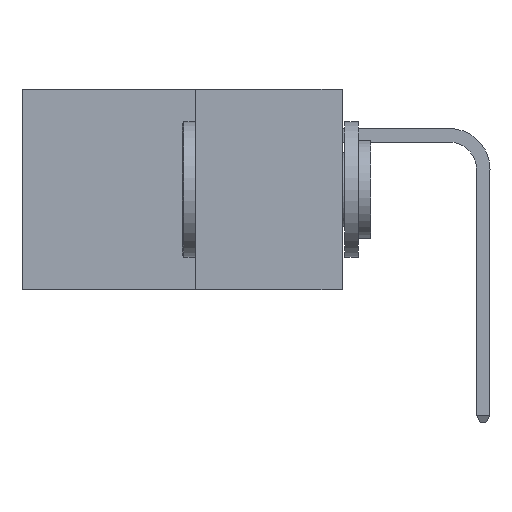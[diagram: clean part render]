
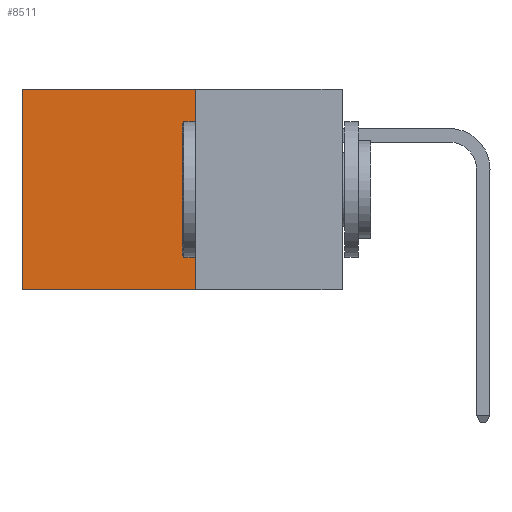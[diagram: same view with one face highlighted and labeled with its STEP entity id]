
A CAD part, left-side view. The second image highlights one B-rep face of the part: STEP entity #8511.
In plain terms, the highlighted planar face has unit normal (-1, 0, 0).
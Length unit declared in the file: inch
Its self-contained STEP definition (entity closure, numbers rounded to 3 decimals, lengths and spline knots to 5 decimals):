
#15 = CARTESIAN_POINT ( 'NONE',  ( 0.277, 0.59, 0. ) ) ;
#224 = VECTOR ( 'NONE', #27878, 39.37008 ) ;
#2352 = CARTESIAN_POINT ( 'NONE',  ( 0.277, 0.27, -0.37 ) ) ;
#2370 = VECTOR ( 'NONE', #6922, 39.37008 ) ;
#2996 = DIRECTION ( 'NONE',  ( 0., 1., 0. ) ) ;
#3148 = CARTESIAN_POINT ( 'NONE',  ( 0.277, 0.27, -0.37 ) ) ;
#3761 = CARTESIAN_POINT ( 'NONE',  ( 0.277, 0.27, -0.37 ) ) ;
#3870 = PLANE ( 'NONE',  #5842 ) ;
#4080 = EDGE_CURVE ( 'NONE', #11165, #22216, #29200, .T. ) ;
#5842 = AXIS2_PLACEMENT_3D ( 'NONE', #3761, #15514, #15857 ) ;
#6637 = EDGE_CURVE ( 'NONE', #14495, #17882, #29067, .T. ) ;
#6922 = DIRECTION ( 'NONE',  ( 0., 0., -1. ) ) ;
#8080 = EDGE_LOOP ( 'NONE', ( #17532, #30637, #21083, #31452 ) ) ;
#8398 = EDGE_CURVE ( 'NONE', #22216, #17882, #28182, .T. ) ;
#8511 = ADVANCED_FACE ( 'NONE', ( #11684 ), #3870, .F. ) ;
#10854 = CARTESIAN_POINT ( 'NONE',  ( 0.277, 0.27, -0.37 ) ) ;
#11165 = VERTEX_POINT ( 'NONE', #13848 ) ;
#11684 = FACE_OUTER_BOUND ( 'NONE', #8080, .T. ) ;
#12030 = EDGE_CURVE ( 'NONE', #11165, #14495, #20380, .T. ) ;
#13848 = CARTESIAN_POINT ( 'NONE',  ( 0.277, 0.27, 0. ) ) ;
#14495 = VERTEX_POINT ( 'NONE', #15 ) ;
#14824 = VECTOR ( 'NONE', #2996, 39.37008 ) ;
#15514 = DIRECTION ( 'NONE',  ( 1., 0., 0. ) ) ;
#15653 = CARTESIAN_POINT ( 'NONE',  ( 0.277, 0.59, -0.37 ) ) ;
#15857 = DIRECTION ( 'NONE',  ( 0., 0., -1. ) ) ;
#16700 = VECTOR ( 'NONE', #23188, 39.37008 ) ;
#17532 = ORIENTED_EDGE ( 'NONE', *, *, #6637, .T. ) ;
#17882 = VERTEX_POINT ( 'NONE', #20454 ) ;
#20380 = LINE ( 'NONE', #30262, #224 ) ;
#20454 = CARTESIAN_POINT ( 'NONE',  ( 0.277, 0.59, -0.37 ) ) ;
#21083 = ORIENTED_EDGE ( 'NONE', *, *, #4080, .F. ) ;
#22216 = VERTEX_POINT ( 'NONE', #2352 ) ;
#23188 = DIRECTION ( 'NONE',  ( 0., 0., -1. ) ) ;
#27878 = DIRECTION ( 'NONE',  ( 0., 1., 0. ) ) ;
#28182 = LINE ( 'NONE', #3148, #14824 ) ;
#29067 = LINE ( 'NONE', #15653, #2370 ) ;
#29200 = LINE ( 'NONE', #10854, #16700 ) ;
#30262 = CARTESIAN_POINT ( 'NONE',  ( 0.277, 0.27, 0. ) ) ;
#30637 = ORIENTED_EDGE ( 'NONE', *, *, #8398, .F. ) ;
#31452 = ORIENTED_EDGE ( 'NONE', *, *, #12030, .T. ) ;
